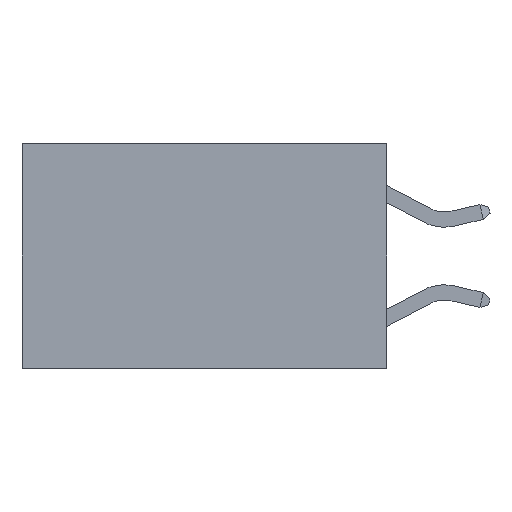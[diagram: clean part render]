
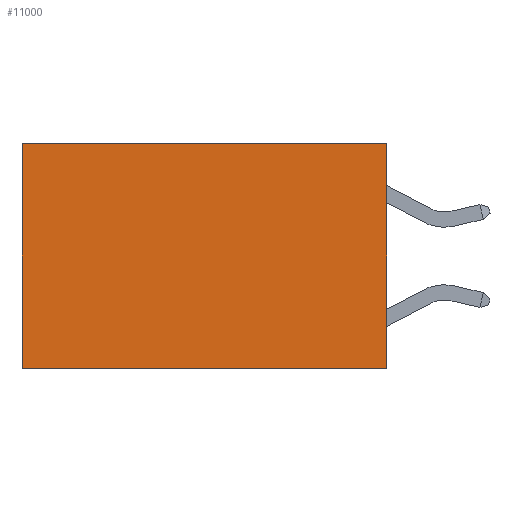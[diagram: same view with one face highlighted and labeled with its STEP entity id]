
A CAD part, left-side view. The second image highlights one B-rep face of the part: STEP entity #11000.
In plain terms, the highlighted planar face has unit normal (-1, 0, 0).
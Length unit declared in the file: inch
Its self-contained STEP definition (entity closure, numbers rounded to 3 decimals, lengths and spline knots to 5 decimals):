
#1090 = DIRECTION ( 'NONE',  ( 0., 1., 0. ) ) ;
#1258 = CARTESIAN_POINT ( 'NONE',  ( 0.2625, 0., 0. ) ) ;
#1412 = CARTESIAN_POINT ( 'NONE',  ( 0.2625, 0., 0. ) ) ;
#1840 = LINE ( 'NONE', #15836, #14923 ) ;
#1896 = ORIENTED_EDGE ( 'NONE', *, *, #14728, .F. ) ;
#2210 = VERTEX_POINT ( 'NONE', #6102 ) ;
#2511 = DIRECTION ( 'NONE',  ( 1., 0., 0. ) ) ;
#3548 = DIRECTION ( 'NONE',  ( 0., 0., -1. ) ) ;
#3980 = DIRECTION ( 'NONE',  ( 0., 0., -1. ) ) ;
#4825 = CARTESIAN_POINT ( 'NONE',  ( 0.2625, 0., -0.37 ) ) ;
#4854 = EDGE_CURVE ( 'NONE', #14739, #2210, #11388, .T. ) ;
#5264 = EDGE_CURVE ( 'NONE', #11092, #12223, #1840, .T. ) ;
#5397 = LINE ( 'NONE', #15743, #14717 ) ;
#5436 = CARTESIAN_POINT ( 'NONE',  ( 0.2625, 0., -0.37 ) ) ;
#5807 = LINE ( 'NONE', #10174, #11552 ) ;
#6102 = CARTESIAN_POINT ( 'NONE',  ( 0.2625, 0.6, -0.37 ) ) ;
#6691 = DIRECTION ( 'NONE',  ( 0., 1., 0. ) ) ;
#7387 = VECTOR ( 'NONE', #6691, 39.37008 ) ;
#8261 = EDGE_LOOP ( 'NONE', ( #9498, #15541, #1896, #14774 ) ) ;
#8651 = AXIS2_PLACEMENT_3D ( 'NONE', #1258, #2511, #11209 ) ;
#9498 = ORIENTED_EDGE ( 'NONE', *, *, #12990, .T. ) ;
#10174 = CARTESIAN_POINT ( 'NONE',  ( 0.2625, 0.6, 0. ) ) ;
#11000 = ADVANCED_FACE ( 'NONE', ( #13284 ), #12373, .F. ) ;
#11092 = VERTEX_POINT ( 'NONE', #1412 ) ;
#11209 = DIRECTION ( 'NONE',  ( 0., 0., -1. ) ) ;
#11388 = LINE ( 'NONE', #5436, #7387 ) ;
#11552 = VECTOR ( 'NONE', #3980, 39.37008 ) ;
#12223 = VERTEX_POINT ( 'NONE', #15745 ) ;
#12373 = PLANE ( 'NONE',  #8651 ) ;
#12990 = EDGE_CURVE ( 'NONE', #12223, #2210, #5807, .T. ) ;
#13284 = FACE_OUTER_BOUND ( 'NONE', #8261, .T. ) ;
#14717 = VECTOR ( 'NONE', #3548, 39.37008 ) ;
#14728 = EDGE_CURVE ( 'NONE', #11092, #14739, #5397, .T. ) ;
#14739 = VERTEX_POINT ( 'NONE', #4825 ) ;
#14774 = ORIENTED_EDGE ( 'NONE', *, *, #5264, .T. ) ;
#14923 = VECTOR ( 'NONE', #1090, 39.37008 ) ;
#15541 = ORIENTED_EDGE ( 'NONE', *, *, #4854, .F. ) ;
#15743 = CARTESIAN_POINT ( 'NONE',  ( 0.2625, 0., 0. ) ) ;
#15745 = CARTESIAN_POINT ( 'NONE',  ( 0.2625, 0.6, 0. ) ) ;
#15836 = CARTESIAN_POINT ( 'NONE',  ( 0.2625, 0., 0. ) ) ;
